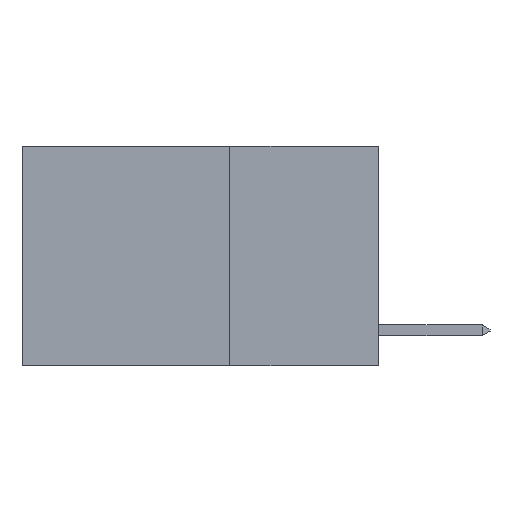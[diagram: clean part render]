
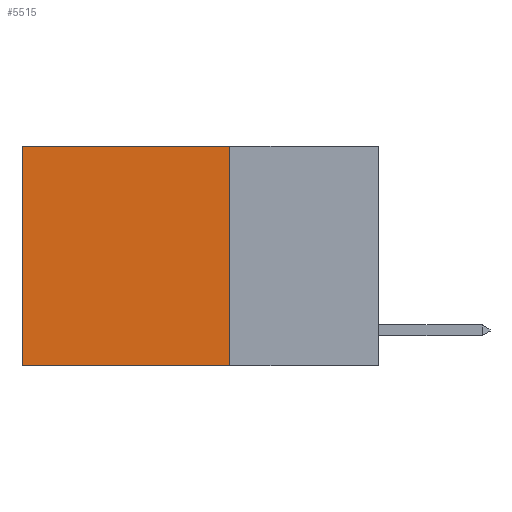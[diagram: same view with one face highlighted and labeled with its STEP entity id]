
A CAD part, left-side view. The second image highlights one B-rep face of the part: STEP entity #5515.
In plain terms, the highlighted planar face has unit normal (-1, 0, 0).
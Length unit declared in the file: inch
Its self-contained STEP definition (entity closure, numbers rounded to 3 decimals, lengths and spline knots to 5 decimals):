
#352 = DIRECTION ( 'NONE',  ( 1., 0., 0. ) ) ;
#371 = CARTESIAN_POINT ( 'NONE',  ( 0.2625, 0.25, -0.37 ) ) ;
#519 = VECTOR ( 'NONE', #7206, 39.37008 ) ;
#677 = AXIS2_PLACEMENT_3D ( 'NONE', #8236, #352, #6027 ) ;
#689 = VECTOR ( 'NONE', #9917, 39.37008 ) ;
#701 = VECTOR ( 'NONE', #2362, 39.37008 ) ;
#704 = CARTESIAN_POINT ( 'NONE',  ( 0.2625, 0.6, 0. ) ) ;
#986 = FACE_OUTER_BOUND ( 'NONE', #1102, .T. ) ;
#1102 = EDGE_LOOP ( 'NONE', ( #3134, #9832, #3077, #3048 ) ) ;
#1560 = CARTESIAN_POINT ( 'NONE',  ( 0.2625, 0.25, 0. ) ) ;
#2362 = DIRECTION ( 'NONE',  ( 0., 1., 0. ) ) ;
#2640 = CARTESIAN_POINT ( 'NONE',  ( 0.2625, 0.25, 0. ) ) ;
#2946 = VERTEX_POINT ( 'NONE', #704 ) ;
#3048 = ORIENTED_EDGE ( 'NONE', *, *, #9393, .T. ) ;
#3077 = ORIENTED_EDGE ( 'NONE', *, *, #5154, .F. ) ;
#3134 = ORIENTED_EDGE ( 'NONE', *, *, #6929, .T. ) ;
#3172 = VERTEX_POINT ( 'NONE', #9726 ) ;
#4784 = LINE ( 'NONE', #10156, #519 ) ;
#4888 = VERTEX_POINT ( 'NONE', #371 ) ;
#4951 = LINE ( 'NONE', #9160, #689 ) ;
#5142 = VERTEX_POINT ( 'NONE', #7453 ) ;
#5154 = EDGE_CURVE ( 'NONE', #5142, #4888, #8431, .T. ) ;
#5187 = PLANE ( 'NONE',  #677 ) ;
#5515 = ADVANCED_FACE ( 'NONE', ( #986 ), #5187, .F. ) ;
#6027 = DIRECTION ( 'NONE',  ( 0., 0., -1. ) ) ;
#6234 = VECTOR ( 'NONE', #8931, 39.37008 ) ;
#6929 = EDGE_CURVE ( 'NONE', #2946, #3172, #4951, .T. ) ;
#7206 = DIRECTION ( 'NONE',  ( 0., 1., 0. ) ) ;
#7453 = CARTESIAN_POINT ( 'NONE',  ( 0.2625, 0.25, 0. ) ) ;
#7744 = EDGE_CURVE ( 'NONE', #4888, #3172, #4784, .T. ) ;
#8236 = CARTESIAN_POINT ( 'NONE',  ( 0.2625, 0.25, 0. ) ) ;
#8431 = LINE ( 'NONE', #2640, #6234 ) ;
#8931 = DIRECTION ( 'NONE',  ( 0., 0., -1. ) ) ;
#9040 = LINE ( 'NONE', #1560, #701 ) ;
#9160 = CARTESIAN_POINT ( 'NONE',  ( 0.2625, 0.6, 0. ) ) ;
#9393 = EDGE_CURVE ( 'NONE', #5142, #2946, #9040, .T. ) ;
#9726 = CARTESIAN_POINT ( 'NONE',  ( 0.2625, 0.6, -0.37 ) ) ;
#9832 = ORIENTED_EDGE ( 'NONE', *, *, #7744, .F. ) ;
#9917 = DIRECTION ( 'NONE',  ( 0., 0., -1. ) ) ;
#10156 = CARTESIAN_POINT ( 'NONE',  ( 0.2625, 0.25, -0.37 ) ) ;
